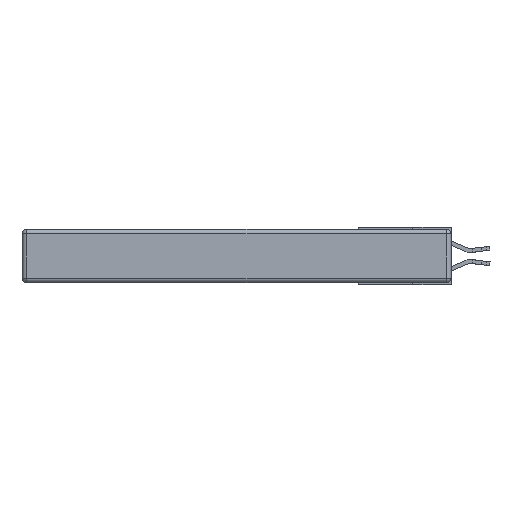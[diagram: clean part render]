
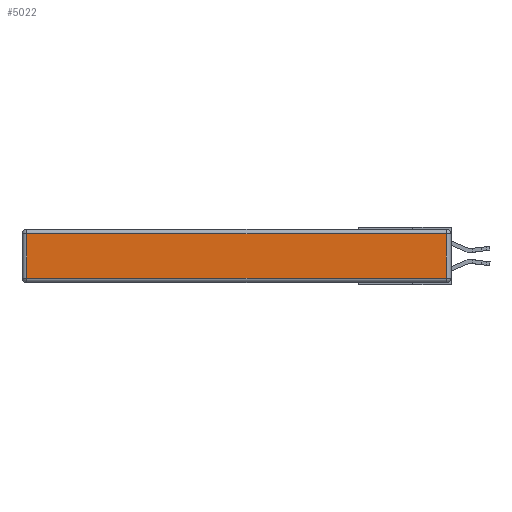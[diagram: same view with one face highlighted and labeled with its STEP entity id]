
A CAD part, left-side view. The second image highlights one B-rep face of the part: STEP entity #5022.
In plain terms, the highlighted planar face has unit normal (-1, 0, 0).
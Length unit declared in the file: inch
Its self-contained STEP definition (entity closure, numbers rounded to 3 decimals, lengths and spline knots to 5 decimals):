
#112 = VERTEX_POINT ( 'NONE', #530 ) ;
#493 = VERTEX_POINT ( 'NONE', #12478 ) ;
#530 = CARTESIAN_POINT ( 'NONE',  ( 0., 0.03, -0.313 ) ) ;
#601 = EDGE_LOOP ( 'NONE', ( #12442, #2470, #11680, #5166 ) ) ;
#690 = CARTESIAN_POINT ( 'NONE',  ( 0., 2.72, -0.03 ) ) ;
#1917 = CARTESIAN_POINT ( 'NONE',  ( 0., 2.72, -0.343 ) ) ;
#2470 = ORIENTED_EDGE ( 'NONE', *, *, #9523, .T. ) ;
#3809 = LINE ( 'NONE', #1917, #13975 ) ;
#3902 = AXIS2_PLACEMENT_3D ( 'NONE', #14347, #8868, #10877 ) ;
#4003 = LINE ( 'NONE', #11967, #13993 ) ;
#4368 = LINE ( 'NONE', #6531, #6717 ) ;
#4937 = EDGE_CURVE ( 'NONE', #493, #112, #4003, .T. ) ;
#5022 = ADVANCED_FACE ( 'NONE', ( #5636 ), #14274, .T. ) ;
#5166 = ORIENTED_EDGE ( 'NONE', *, *, #10096, .T. ) ;
#5636 = FACE_OUTER_BOUND ( 'NONE', #601, .T. ) ;
#6531 = CARTESIAN_POINT ( 'NONE',  ( 0., 0.03, -0.343 ) ) ;
#6717 = VECTOR ( 'NONE', #11368, 39.37008 ) ;
#6736 = VERTEX_POINT ( 'NONE', #12290 ) ;
#8419 = VERTEX_POINT ( 'NONE', #690 ) ;
#8716 = LINE ( 'NONE', #14168, #11465 ) ;
#8868 = DIRECTION ( 'NONE',  ( -1., 0., 0. ) ) ;
#9358 = EDGE_CURVE ( 'NONE', #6736, #8419, #8716, .T. ) ;
#9523 = EDGE_CURVE ( 'NONE', #112, #6736, #4368, .T. ) ;
#9845 = DIRECTION ( 'NONE',  ( 0., 0., -1. ) ) ;
#10096 = EDGE_CURVE ( 'NONE', #8419, #493, #3809, .T. ) ;
#10877 = DIRECTION ( 'NONE',  ( 0., 0., 1. ) ) ;
#11368 = DIRECTION ( 'NONE',  ( 0., 0., 1. ) ) ;
#11465 = VECTOR ( 'NONE', #12955, 39.37008 ) ;
#11680 = ORIENTED_EDGE ( 'NONE', *, *, #9358, .T. ) ;
#11967 = CARTESIAN_POINT ( 'NONE',  ( 0., 0., -0.313 ) ) ;
#12290 = CARTESIAN_POINT ( 'NONE',  ( 0., 0.03, -0.03 ) ) ;
#12442 = ORIENTED_EDGE ( 'NONE', *, *, #4937, .T. ) ;
#12478 = CARTESIAN_POINT ( 'NONE',  ( 0., 2.72, -0.313 ) ) ;
#12955 = DIRECTION ( 'NONE',  ( 0., 1., 0. ) ) ;
#13975 = VECTOR ( 'NONE', #9845, 39.37008 ) ;
#13993 = VECTOR ( 'NONE', #14171, 39.37008 ) ;
#14168 = CARTESIAN_POINT ( 'NONE',  ( 0., 2.75, -0.03 ) ) ;
#14171 = DIRECTION ( 'NONE',  ( 0., -1., 0. ) ) ;
#14274 = PLANE ( 'NONE',  #3902 ) ;
#14347 = CARTESIAN_POINT ( 'NONE',  ( 0., 0., -0.343 ) ) ;
